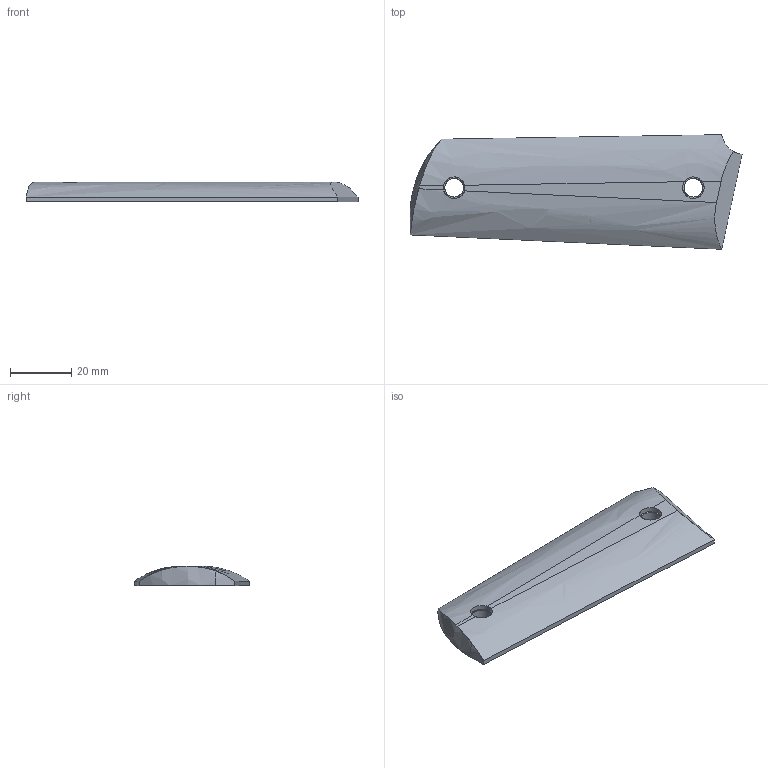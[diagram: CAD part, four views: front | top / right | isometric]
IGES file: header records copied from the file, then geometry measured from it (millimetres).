
Global section: file name: 1911_grips_blank_left.igs; native system: GibbsCAM 8.0.28 NLO; preprocessor: Exchange 1.0; author: dumpster; organization: dcnc; date: 070215.232801; units: inch
Bounding box: 108.39 x 37.39 x 6.35 mm (x, y, z)
Surface area: 7942.4 mm2 (no closed solid volume)
Topology: 0 solids, 0 shells, 22 faces, 345 edges, 343 vertices
Faces by surface type: bspline 22
